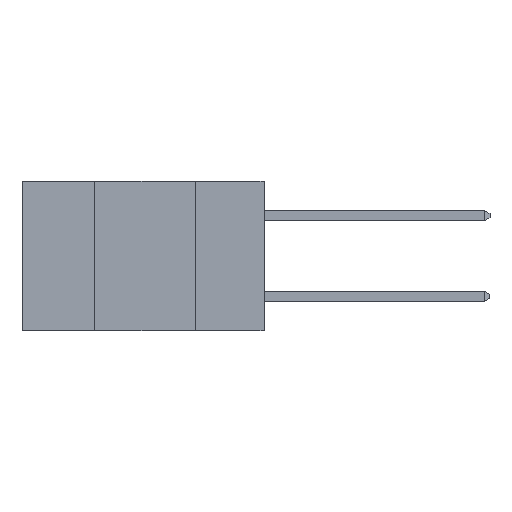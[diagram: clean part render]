
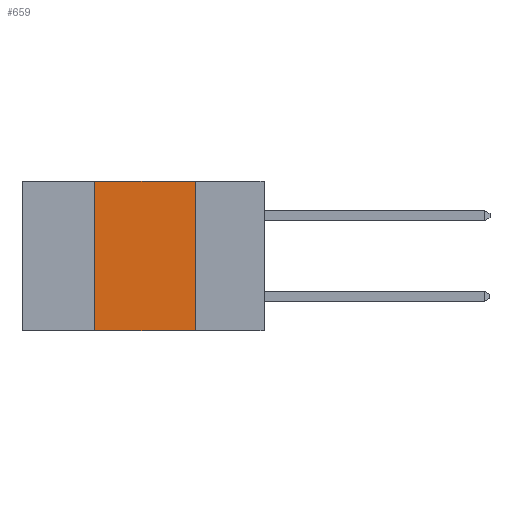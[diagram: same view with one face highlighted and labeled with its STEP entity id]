
A CAD part, left-side view. The second image highlights one B-rep face of the part: STEP entity #659.
In plain terms, the highlighted planar face has unit normal (-1, 0, 0).
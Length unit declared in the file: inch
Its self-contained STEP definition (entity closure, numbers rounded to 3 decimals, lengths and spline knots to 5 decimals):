
#42 = CARTESIAN_POINT ( 'NONE',  ( 0., 0.17, 0. ) ) ;
#659 = ADVANCED_FACE ( 'NONE', ( #17496 ), #16283, .F. ) ;
#1218 = LINE ( 'NONE', #14671, #8779 ) ;
#2146 = DIRECTION ( 'NONE',  ( 0., 0., 1. ) ) ;
#2164 = CARTESIAN_POINT ( 'NONE',  ( 0., 0.17, -0.37 ) ) ;
#3034 = ORIENTED_EDGE ( 'NONE', *, *, #4743, .F. ) ;
#3407 = LINE ( 'NONE', #8177, #18057 ) ;
#3824 = ORIENTED_EDGE ( 'NONE', *, *, #11146, .T. ) ;
#3999 = CARTESIAN_POINT ( 'NONE',  ( 0., 0.6, -0.37 ) ) ;
#4743 = EDGE_CURVE ( 'NONE', #6000, #16976, #7864, .T. ) ;
#6000 = VERTEX_POINT ( 'NONE', #6982 ) ;
#6060 = AXIS2_PLACEMENT_3D ( 'NONE', #8182, #16043, #13573 ) ;
#6459 = LINE ( 'NONE', #3999, #13230 ) ;
#6982 = CARTESIAN_POINT ( 'NONE',  ( 0., 0.17, 0. ) ) ;
#7864 = LINE ( 'NONE', #42, #11231 ) ;
#8177 = CARTESIAN_POINT ( 'NONE',  ( 0., 0.42, 0. ) ) ;
#8182 = CARTESIAN_POINT ( 'NONE',  ( 0., 0.6, 0. ) ) ;
#8506 = DIRECTION ( 'NONE',  ( 0., -1., 0. ) ) ;
#8590 = VERTEX_POINT ( 'NONE', #13652 ) ;
#8779 = VECTOR ( 'NONE', #13272, 39.37008 ) ;
#8838 = DIRECTION ( 'NONE',  ( 0., 0., -1. ) ) ;
#9375 = EDGE_LOOP ( 'NONE', ( #3034, #11742, #11237, #3824 ) ) ;
#10752 = CARTESIAN_POINT ( 'NONE',  ( 0., 0.42, 0. ) ) ;
#11146 = EDGE_CURVE ( 'NONE', #8590, #16976, #6459, .T. ) ;
#11231 = VECTOR ( 'NONE', #8838, 39.37008 ) ;
#11237 = ORIENTED_EDGE ( 'NONE', *, *, #15737, .F. ) ;
#11742 = ORIENTED_EDGE ( 'NONE', *, *, #16062, .F. ) ;
#13230 = VECTOR ( 'NONE', #8506, 39.37008 ) ;
#13272 = DIRECTION ( 'NONE',  ( 0., -1., 0. ) ) ;
#13573 = DIRECTION ( 'NONE',  ( 0., 0., -1. ) ) ;
#13652 = CARTESIAN_POINT ( 'NONE',  ( 0., 0.42, -0.37 ) ) ;
#14671 = CARTESIAN_POINT ( 'NONE',  ( 0., 0.6, 0. ) ) ;
#15737 = EDGE_CURVE ( 'NONE', #8590, #17515, #3407, .T. ) ;
#16043 = DIRECTION ( 'NONE',  ( 1., 0., 0. ) ) ;
#16062 = EDGE_CURVE ( 'NONE', #17515, #6000, #1218, .T. ) ;
#16283 = PLANE ( 'NONE',  #6060 ) ;
#16976 = VERTEX_POINT ( 'NONE', #2164 ) ;
#17496 = FACE_OUTER_BOUND ( 'NONE', #9375, .T. ) ;
#17515 = VERTEX_POINT ( 'NONE', #10752 ) ;
#18057 = VECTOR ( 'NONE', #2146, 39.37008 ) ;
